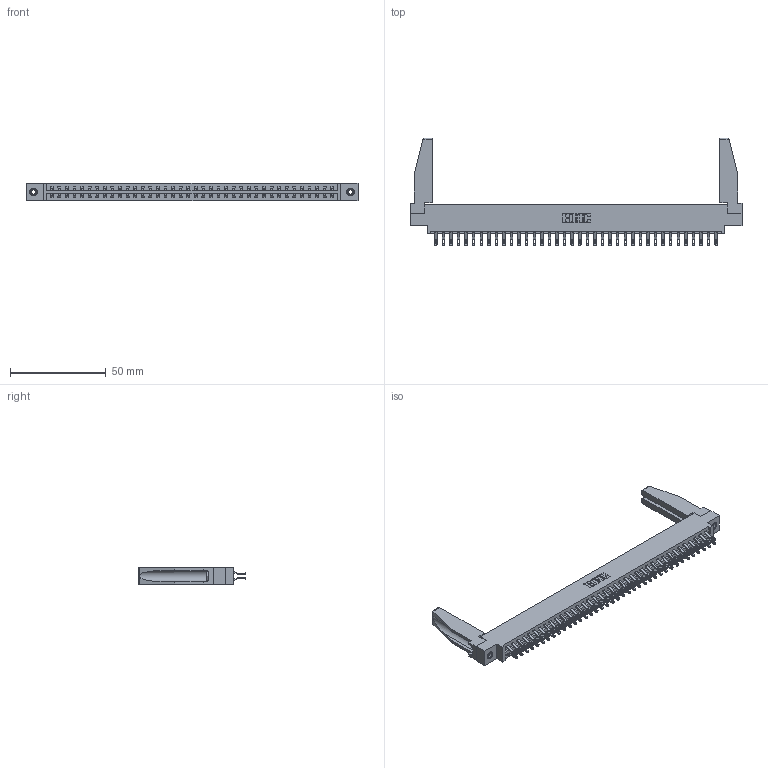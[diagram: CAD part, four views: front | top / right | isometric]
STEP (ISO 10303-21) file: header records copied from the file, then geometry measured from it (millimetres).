
FILE_DESCRIPTION (( 'STEP AP203' ), '1' );
FILE_NAME ('337-076-555-878.STEP', '2019-10-15T13:37:10', ( '' ), ( '' ), 'SwSTEP 2.0', 'SolidWorks 2016', '' );
FILE_SCHEMA (( 'CONFIG_CONTROL_DESIGN' ));
Length unit declared in the file: inch
Products named in the file (5): 307-220-078; 337-076-555-878; 337 Part_0.170 Offset - 0.156 Dia-TI; 345-250-001_345-250-001-102; 345-292-001_555 Tail
Assembly tree (81 placements, depth 2):
  337-076-555-878
    337 Part_0.170 Offset - 0.156 Dia-TI
    345-292-001_555 Tail  x76
    345-250-001_345-250-001-102  x2
    307-220-078  x2
Bounding box: 173.58 x 56.27 x 9.4 mm (x, y, z)
Volume: 22336.6 mm3; surface area: 25467.3 mm2
Topology: 81 solids, 81 shells, 4808 faces, 15017 edges, 10002 vertices
Faces by surface type: plane 2894, cylinder 1898, cone 12, torus 4
Entity records: 32878 total; most frequent: CARTESIAN_POINT 5578, ORIENTED_EDGE 5440, DIRECTION 4728, EDGE_CURVE 2720, LINE 2534, VECTOR 2534, VERTEX_POINT 1808, AXIS2_PLACEMENT_3D 1097
